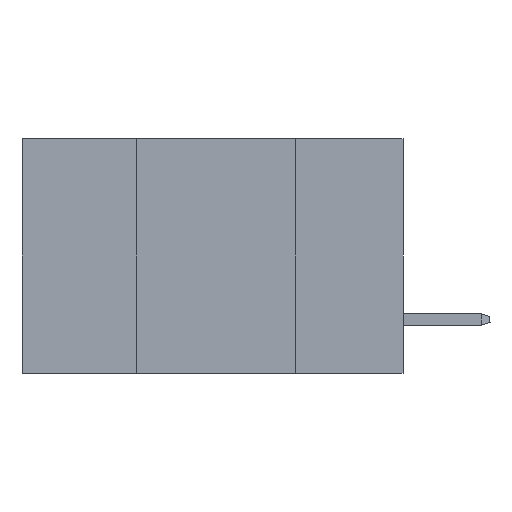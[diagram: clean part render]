
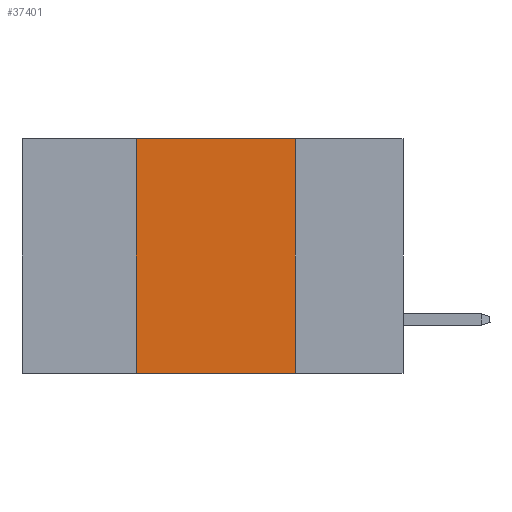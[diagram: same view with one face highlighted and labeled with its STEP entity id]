
A CAD part, left-side view. The second image highlights one B-rep face of the part: STEP entity #37401.
In plain terms, the highlighted planar face has unit normal (-1, 0, 0).
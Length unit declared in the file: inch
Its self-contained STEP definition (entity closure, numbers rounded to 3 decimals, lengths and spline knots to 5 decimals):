
#1052 = VECTOR ( 'NONE', #16586, 39.37008 ) ;
#1224 = EDGE_CURVE ( 'NONE', #16397, #38667, #23342, .T. ) ;
#3535 = LINE ( 'NONE', #10034, #29227 ) ;
#6342 = CARTESIAN_POINT ( 'NONE',  ( 0., 0.42, -0.37 ) ) ;
#6531 = DIRECTION ( 'NONE',  ( 1., 0., 0. ) ) ;
#9188 = VECTOR ( 'NONE', #43781, 39.37008 ) ;
#9319 = EDGE_CURVE ( 'NONE', #26647, #16397, #44279, .T. ) ;
#10034 = CARTESIAN_POINT ( 'NONE',  ( 0., 0.6, -0.37 ) ) ;
#11645 = DIRECTION ( 'NONE',  ( 0., 0., 1. ) ) ;
#12094 = CARTESIAN_POINT ( 'NONE',  ( 0., 0.17, 0. ) ) ;
#12346 = CARTESIAN_POINT ( 'NONE',  ( 0., 0.42, 0. ) ) ;
#15320 = VERTEX_POINT ( 'NONE', #36819 ) ;
#16397 = VERTEX_POINT ( 'NONE', #16934 ) ;
#16586 = DIRECTION ( 'NONE',  ( 0., -1., 0. ) ) ;
#16934 = CARTESIAN_POINT ( 'NONE',  ( 0., 0.42, 0. ) ) ;
#17229 = PLANE ( 'NONE',  #21860 ) ;
#21860 = AXIS2_PLACEMENT_3D ( 'NONE', #24223, #6531, #34928 ) ;
#22242 = ORIENTED_EDGE ( 'NONE', *, *, #9319, .F. ) ;
#23342 = LINE ( 'NONE', #34742, #1052 ) ;
#24223 = CARTESIAN_POINT ( 'NONE',  ( 0., 0.6, 0. ) ) ;
#24420 = EDGE_LOOP ( 'NONE', ( #40755, #45059, #22242, #37137 ) ) ;
#26647 = VERTEX_POINT ( 'NONE', #6342 ) ;
#27514 = DIRECTION ( 'NONE',  ( 0., -1., 0. ) ) ;
#29227 = VECTOR ( 'NONE', #27514, 39.37008 ) ;
#30179 = EDGE_CURVE ( 'NONE', #38667, #15320, #44256, .T. ) ;
#34742 = CARTESIAN_POINT ( 'NONE',  ( 0., 0.6, 0. ) ) ;
#34928 = DIRECTION ( 'NONE',  ( 0., 0., -1. ) ) ;
#36557 = EDGE_CURVE ( 'NONE', #26647, #15320, #3535, .T. ) ;
#36819 = CARTESIAN_POINT ( 'NONE',  ( 0., 0.17, -0.37 ) ) ;
#37137 = ORIENTED_EDGE ( 'NONE', *, *, #36557, .T. ) ;
#37401 = ADVANCED_FACE ( 'NONE', ( #41894 ), #17229, .F. ) ;
#38667 = VERTEX_POINT ( 'NONE', #44003 ) ;
#40755 = ORIENTED_EDGE ( 'NONE', *, *, #30179, .F. ) ;
#41190 = VECTOR ( 'NONE', #11645, 39.37008 ) ;
#41894 = FACE_OUTER_BOUND ( 'NONE', #24420, .T. ) ;
#43781 = DIRECTION ( 'NONE',  ( 0., 0., -1. ) ) ;
#44003 = CARTESIAN_POINT ( 'NONE',  ( 0., 0.17, 0. ) ) ;
#44256 = LINE ( 'NONE', #12094, #9188 ) ;
#44279 = LINE ( 'NONE', #12346, #41190 ) ;
#45059 = ORIENTED_EDGE ( 'NONE', *, *, #1224, .F. ) ;
